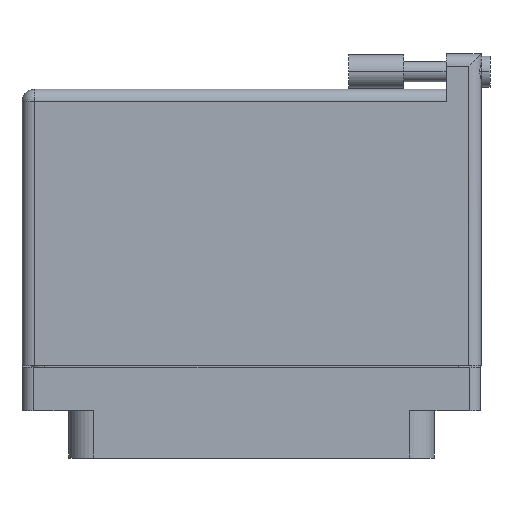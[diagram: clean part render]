
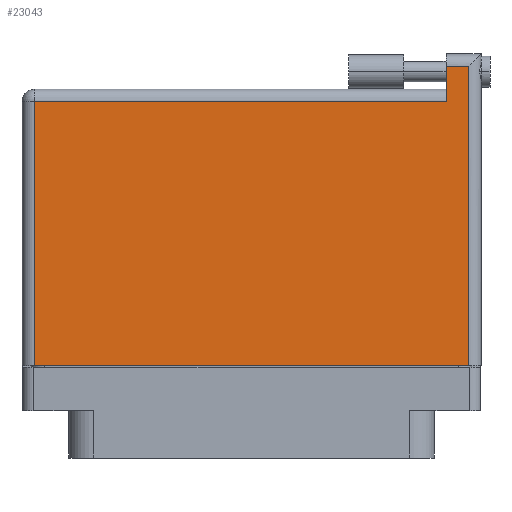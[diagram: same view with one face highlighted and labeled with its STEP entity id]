
A CAD part, front view. The second image highlights one B-rep face of the part: STEP entity #23043.
In plain terms, the highlighted face is planar.
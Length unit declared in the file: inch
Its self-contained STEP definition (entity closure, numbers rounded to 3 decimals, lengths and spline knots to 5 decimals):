
#1124 = ORIENTED_EDGE ( 'NONE', *, *, #29692, .T. ) ;
#1352 = DIRECTION ( 'NONE',  ( -1., 0., 0. ) ) ;
#2742 = PLANE ( 'NONE',  #32539 ) ;
#2836 = VERTEX_POINT ( 'NONE', #17779 ) ;
#4689 = EDGE_CURVE ( 'NONE', #36708, #44303, #13878, .T. ) ;
#5507 = EDGE_CURVE ( 'NONE', #20155, #30785, #13221, .T. ) ;
#5805 = DIRECTION ( 'NONE',  ( 0., -1., 0. ) ) ;
#5876 = DIRECTION ( 'NONE',  ( -1., 0., 0. ) ) ;
#6109 = LINE ( 'NONE', #34260, #24025 ) ;
#6840 = EDGE_CURVE ( 'NONE', #30785, #25808, #17078, .T. ) ;
#8483 = ORIENTED_EDGE ( 'NONE', *, *, #5507, .T. ) ;
#8915 = ORIENTED_EDGE ( 'NONE', *, *, #6840, .T. ) ;
#9581 = VECTOR ( 'NONE', #26617, 39.37008 ) ;
#10798 = DIRECTION ( 'NONE',  ( 0., 1., 0. ) ) ;
#11251 = EDGE_CURVE ( 'NONE', #25808, #36708, #29448, .T. ) ;
#12875 = ORIENTED_EDGE ( 'NONE', *, *, #4689, .T. ) ;
#12894 = CARTESIAN_POINT ( 'NONE',  ( -1.3, 1.596, 0.4495 ) ) ;
#13221 = LINE ( 'NONE', #12894, #46175 ) ;
#13878 = LINE ( 'NONE', #31338, #25488 ) ;
#17078 = LINE ( 'NONE', #34420, #9581 ) ;
#17779 = CARTESIAN_POINT ( 'NONE',  ( 1.23, -0.1, 0.4495 ) ) ;
#19261 = CARTESIAN_POINT ( 'NONE',  ( -1.23, 1.396, 0.4495 ) ) ;
#20155 = VERTEX_POINT ( 'NONE', #47632 ) ;
#20318 = LINE ( 'NONE', #27820, #41733 ) ;
#23043 = ADVANCED_FACE ( 'NONE', ( #45843 ), #2742, .F. ) ;
#23196 = DIRECTION ( 'NONE',  ( 1., 0., 0. ) ) ;
#24025 = VECTOR ( 'NONE', #23196, 39.37008 ) ;
#24139 = CARTESIAN_POINT ( 'NONE',  ( 1.103, 1.396, 0.4495 ) ) ;
#25488 = VECTOR ( 'NONE', #5805, 39.37008 ) ;
#25808 = VERTEX_POINT ( 'NONE', #24139 ) ;
#26617 = DIRECTION ( 'NONE',  ( 0., -1., 0. ) ) ;
#27820 = CARTESIAN_POINT ( 'NONE',  ( 1.23, 1.666, 0.4495 ) ) ;
#28043 = EDGE_LOOP ( 'NONE', ( #1124, #37625, #8483, #8915, #39117, #12875 ) ) ;
#29448 = LINE ( 'NONE', #35775, #46718 ) ;
#29692 = EDGE_CURVE ( 'NONE', #44303, #2836, #6109, .T. ) ;
#30785 = VERTEX_POINT ( 'NONE', #39320 ) ;
#31338 = CARTESIAN_POINT ( 'NONE',  ( -1.23, -0.1, 0.4495 ) ) ;
#32279 = CARTESIAN_POINT ( 'NONE',  ( -1.3, 1.466, 0.4495 ) ) ;
#32539 = AXIS2_PLACEMENT_3D ( 'NONE', #32279, #39714, #47030 ) ;
#34260 = CARTESIAN_POINT ( 'NONE',  ( -1.3, -0.1, 0.4495 ) ) ;
#34420 = CARTESIAN_POINT ( 'NONE',  ( 1.103, 1.666, 0.4495 ) ) ;
#34980 = CARTESIAN_POINT ( 'NONE',  ( -1.23, -0.1, 0.4495 ) ) ;
#35775 = CARTESIAN_POINT ( 'NONE',  ( -1.3, 1.396, 0.4495 ) ) ;
#36708 = VERTEX_POINT ( 'NONE', #19261 ) ;
#37625 = ORIENTED_EDGE ( 'NONE', *, *, #46262, .T. ) ;
#39117 = ORIENTED_EDGE ( 'NONE', *, *, #11251, .T. ) ;
#39320 = CARTESIAN_POINT ( 'NONE',  ( 1.103, 1.596, 0.4495 ) ) ;
#39714 = DIRECTION ( 'NONE',  ( 0., 0., -1. ) ) ;
#41733 = VECTOR ( 'NONE', #10798, 39.37008 ) ;
#44303 = VERTEX_POINT ( 'NONE', #34980 ) ;
#45843 = FACE_OUTER_BOUND ( 'NONE', #28043, .T. ) ;
#46175 = VECTOR ( 'NONE', #1352, 39.37008 ) ;
#46262 = EDGE_CURVE ( 'NONE', #2836, #20155, #20318, .T. ) ;
#46718 = VECTOR ( 'NONE', #5876, 39.37008 ) ;
#47030 = DIRECTION ( 'NONE',  ( -1., 0., 0. ) ) ;
#47632 = CARTESIAN_POINT ( 'NONE',  ( 1.23, 1.596, 0.4495 ) ) ;
